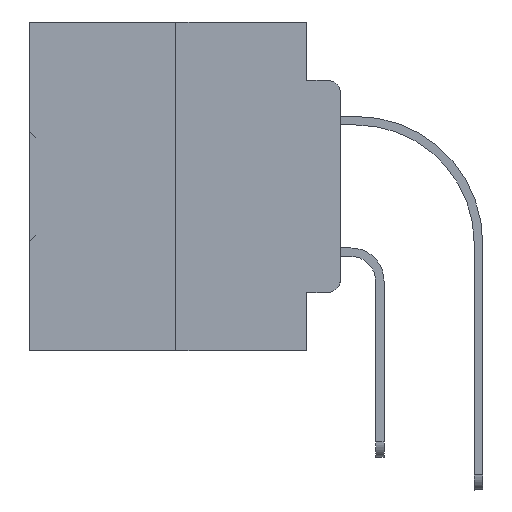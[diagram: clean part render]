
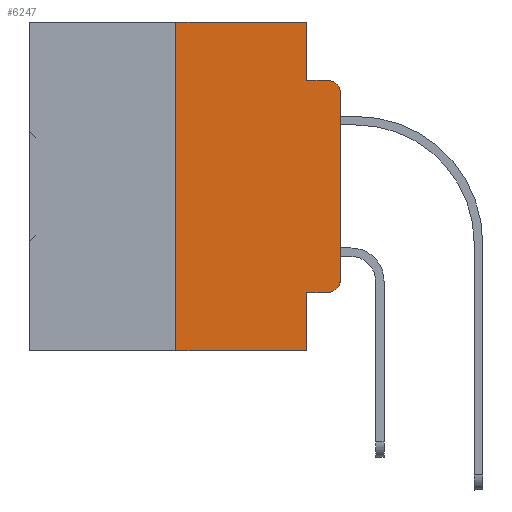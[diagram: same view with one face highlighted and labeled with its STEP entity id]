
A CAD part, left-side view. The second image highlights one B-rep face of the part: STEP entity #6247.
In plain terms, the highlighted planar face has unit normal (-1, 0, 0).
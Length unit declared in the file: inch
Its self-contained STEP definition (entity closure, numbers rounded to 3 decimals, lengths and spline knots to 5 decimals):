
#136 = CARTESIAN_POINT ( 'NONE',  ( 0., 0.25, 0. ) ) ;
#373 = EDGE_CURVE ( 'NONE', #9705, #14305, #2814, .T. ) ;
#478 = CARTESIAN_POINT ( 'NONE',  ( 0., 0.051, 0. ) ) ;
#765 = CARTESIAN_POINT ( 'NONE',  ( 0., 0.25, -0.5 ) ) ;
#893 = AXIS2_PLACEMENT_3D ( 'NONE', #14929, #35978, #35184 ) ;
#945 = VERTEX_POINT ( 'NONE', #765 ) ;
#1369 = ORIENTED_EDGE ( 'NONE', *, *, #10177, .T. ) ;
#2180 = EDGE_CURVE ( 'NONE', #37045, #18086, #29757, .T. ) ;
#2814 = LINE ( 'NONE', #23421, #24647 ) ;
#2889 = DIRECTION ( 'NONE',  ( 0., -1., 0. ) ) ;
#2993 = ORIENTED_EDGE ( 'NONE', *, *, #9325, .F. ) ;
#3263 = DIRECTION ( 'NONE',  ( 0., -1., 0. ) ) ;
#3320 = DIRECTION ( 'NONE',  ( -1., 0., 0. ) ) ;
#4919 = EDGE_CURVE ( 'NONE', #12932, #19470, #16132, .T. ) ;
#5360 = CARTESIAN_POINT ( 'NONE',  ( 0., 0.051, -0.4115 ) ) ;
#5435 = LINE ( 'NONE', #32951, #25992 ) ;
#5796 = VERTEX_POINT ( 'NONE', #31166 ) ;
#6247 = ADVANCED_FACE ( 'NONE', ( #37042 ), #21502, .F. ) ;
#6571 = DIRECTION ( 'NONE',  ( 0., 0., -1. ) ) ;
#7139 = CARTESIAN_POINT ( 'NONE',  ( 0., 0.473, 0. ) ) ;
#9015 = CARTESIAN_POINT ( 'NONE',  ( 0., 0.02, -0.3915 ) ) ;
#9325 = EDGE_CURVE ( 'NONE', #14305, #18086, #5435, .T. ) ;
#9694 = DIRECTION ( 'NONE',  ( 0., 0., -1. ) ) ;
#9705 = VERTEX_POINT ( 'NONE', #11999 ) ;
#10088 = DIRECTION ( 'NONE',  ( 1., 0., 0. ) ) ;
#10173 = VECTOR ( 'NONE', #37565, 39.37008 ) ;
#10177 = EDGE_CURVE ( 'NONE', #19470, #19149, #19146, .T. ) ;
#10428 = CARTESIAN_POINT ( 'NONE',  ( 0., 0.051, -0.4115 ) ) ;
#10435 = LINE ( 'NONE', #28311, #27604 ) ;
#10863 = ORIENTED_EDGE ( 'NONE', *, *, #32952, .T. ) ;
#11841 = ORIENTED_EDGE ( 'NONE', *, *, #14385, .F. ) ;
#11999 = CARTESIAN_POINT ( 'NONE',  ( 0., 0.051, 0. ) ) ;
#12084 = LINE ( 'NONE', #33142, #35048 ) ;
#12548 = ORIENTED_EDGE ( 'NONE', *, *, #4919, .T. ) ;
#12587 = EDGE_CURVE ( 'NONE', #19149, #37045, #32875, .T. ) ;
#12932 = VERTEX_POINT ( 'NONE', #5360 ) ;
#14113 = AXIS2_PLACEMENT_3D ( 'NONE', #9015, #3320, #14903 ) ;
#14305 = VERTEX_POINT ( 'NONE', #31074 ) ;
#14385 = EDGE_CURVE ( 'NONE', #5796, #9705, #10435, .T. ) ;
#14675 = VERTEX_POINT ( 'NONE', #17303 ) ;
#14903 = DIRECTION ( 'NONE',  ( 0., 0., -1. ) ) ;
#14929 = CARTESIAN_POINT ( 'NONE',  ( 0., 0.02, -0.1085 ) ) ;
#15657 = ORIENTED_EDGE ( 'NONE', *, *, #23294, .F. ) ;
#16132 = LINE ( 'NONE', #10428, #10173 ) ;
#17303 = CARTESIAN_POINT ( 'NONE',  ( 0., 0.051, -0.5 ) ) ;
#17715 = CARTESIAN_POINT ( 'NONE',  ( 0., 0., -0.3915 ) ) ;
#17821 = DIRECTION ( 'NONE',  ( 0., 0., 1. ) ) ;
#17925 = DIRECTION ( 'NONE',  ( 0., 0., -1. ) ) ;
#18086 = VERTEX_POINT ( 'NONE', #28421 ) ;
#19146 = CIRCLE ( 'NONE', #14113, 0.02 ) ;
#19149 = VERTEX_POINT ( 'NONE', #17715 ) ;
#19326 = AXIS2_PLACEMENT_3D ( 'NONE', #7139, #10088, #6571 ) ;
#19470 = VERTEX_POINT ( 'NONE', #25862 ) ;
#20282 = DIRECTION ( 'NONE',  ( 0., 0., 1. ) ) ;
#20573 = LINE ( 'NONE', #136, #38671 ) ;
#21502 = PLANE ( 'NONE',  #19326 ) ;
#22615 = CARTESIAN_POINT ( 'NONE',  ( 0., 0., -0.1085 ) ) ;
#22787 = ORIENTED_EDGE ( 'NONE', *, *, #373, .F. ) ;
#23294 = EDGE_CURVE ( 'NONE', #12932, #14675, #24615, .T. ) ;
#23421 = CARTESIAN_POINT ( 'NONE',  ( 0., 0.051, 0. ) ) ;
#23999 = CARTESIAN_POINT ( 'NONE',  ( 0., 0., 0. ) ) ;
#24615 = LINE ( 'NONE', #478, #38472 ) ;
#24647 = VECTOR ( 'NONE', #17925, 39.37008 ) ;
#25555 = VECTOR ( 'NONE', #20282, 39.37008 ) ;
#25862 = CARTESIAN_POINT ( 'NONE',  ( 0., 0.02, -0.4115 ) ) ;
#25992 = VECTOR ( 'NONE', #2889, 39.37008 ) ;
#26251 = EDGE_LOOP ( 'NONE', ( #37736, #35149, #2993, #22787, #11841, #30788, #10863, #15657, #12548, #1369 ) ) ;
#27604 = VECTOR ( 'NONE', #34425, 39.37008 ) ;
#28104 = EDGE_CURVE ( 'NONE', #945, #5796, #20573, .T. ) ;
#28311 = CARTESIAN_POINT ( 'NONE',  ( 0., 0.473, 0. ) ) ;
#28421 = CARTESIAN_POINT ( 'NONE',  ( 0., 0.02, -0.0885 ) ) ;
#29757 = CIRCLE ( 'NONE', #893, 0.02 ) ;
#30788 = ORIENTED_EDGE ( 'NONE', *, *, #28104, .F. ) ;
#31074 = CARTESIAN_POINT ( 'NONE',  ( 0., 0.051, -0.0885 ) ) ;
#31166 = CARTESIAN_POINT ( 'NONE',  ( 0., 0.25, 0. ) ) ;
#32875 = LINE ( 'NONE', #23999, #25555 ) ;
#32951 = CARTESIAN_POINT ( 'NONE',  ( 0., 0.051, -0.0885 ) ) ;
#32952 = EDGE_CURVE ( 'NONE', #945, #14675, #12084, .T. ) ;
#33142 = CARTESIAN_POINT ( 'NONE',  ( 0., 0.473, -0.5 ) ) ;
#34425 = DIRECTION ( 'NONE',  ( 0., -1., 0. ) ) ;
#35048 = VECTOR ( 'NONE', #3263, 39.37008 ) ;
#35149 = ORIENTED_EDGE ( 'NONE', *, *, #2180, .T. ) ;
#35184 = DIRECTION ( 'NONE',  ( 0., 0., -1. ) ) ;
#35978 = DIRECTION ( 'NONE',  ( -1., 0., 0. ) ) ;
#37042 = FACE_OUTER_BOUND ( 'NONE', #26251, .T. ) ;
#37045 = VERTEX_POINT ( 'NONE', #22615 ) ;
#37565 = DIRECTION ( 'NONE',  ( 0., -1., 0. ) ) ;
#37736 = ORIENTED_EDGE ( 'NONE', *, *, #12587, .T. ) ;
#38472 = VECTOR ( 'NONE', #9694, 39.37008 ) ;
#38671 = VECTOR ( 'NONE', #17821, 39.37008 ) ;
